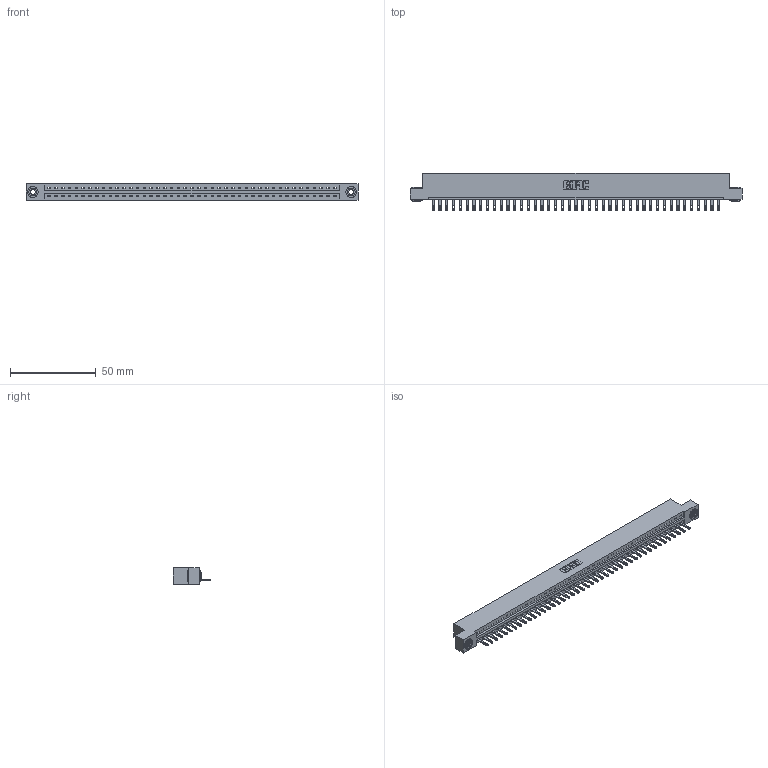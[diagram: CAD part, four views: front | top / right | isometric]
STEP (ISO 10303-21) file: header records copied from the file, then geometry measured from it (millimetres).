
FILE_DESCRIPTION (( 'STEP AP203' ), '1' );
FILE_NAME ('337-043-500-103.STEP', '2018-08-09T02:20:14', ( '' ), ( '' ), 'SwSTEP 2.0', 'SolidWorks 2016', '' );
FILE_SCHEMA (( 'CONFIG_CONTROL_DESIGN' ));
Length unit declared in the file: inch
Products named in the file (4): 337-043-500-103; 337 Part_Flush Mounting Lugs - 0.156 Dia-TH; 345-292-001_345-293-100; 345-250-002_345-250-002-102
Assembly tree (46 placements, depth 2):
  337-043-500-103
    337 Part_Flush Mounting Lugs - 0.156 Dia-TH
    345-292-001_345-293-100  x43
    345-250-002_345-250-002-102  x2
Bounding box: 193.4 x 21.85 x 9.4 mm (x, y, z)
Volume: 20158.7 mm3; surface area: 21169.7 mm2
Topology: 46 solids, 46 shells, 2646 faces, 8127 edges, 5414 vertices
Faces by surface type: plane 1800, cylinder 838, cone 8
Entity records: 32414 total; most frequent: CARTESIAN_POINT 5622, ORIENTED_EDGE 5594, DIRECTION 4765, EDGE_CURVE 2797, LINE 2641, VECTOR 2641, VERTEX_POINT 1862, AXIS2_PLACEMENT_3D 1062
